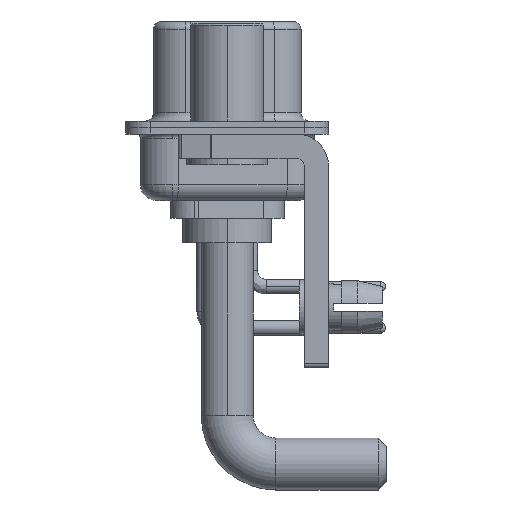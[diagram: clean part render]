
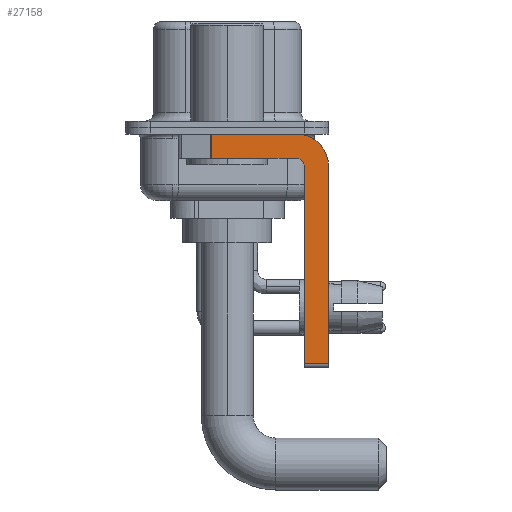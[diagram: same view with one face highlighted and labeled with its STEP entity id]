
A CAD part, left-side view. The second image highlights one B-rep face of the part: STEP entity #27158.
In plain terms, the highlighted planar face has unit normal (-1, 0, 0).
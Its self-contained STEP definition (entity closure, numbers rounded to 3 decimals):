
#80 = AXIS2_PLACEMENT_3D ( 'NONE', #9744, #21357, #2377 ) ;
#564 = VERTEX_POINT ( 'NONE', #26836 ) ;
#746 = VERTEX_POINT ( 'NONE', #25038 ) ;
#824 = DIRECTION ( 'NONE',  ( 0., 0., 1. ) ) ;
#880 = DIRECTION ( 'NONE',  ( 1., 0., 0. ) ) ;
#1668 = CARTESIAN_POINT ( 'NONE',  ( -2.9, -4.75, -14.55 ) ) ;
#2377 = DIRECTION ( 'NONE',  ( 0., 0., -1. ) ) ;
#2420 = DIRECTION ( 'NONE',  ( 0., 0., 1. ) ) ;
#3347 = CARTESIAN_POINT ( 'NONE',  ( -2.9, -6.25, -2.4 ) ) ;
#4554 = LINE ( 'NONE', #18276, #5144 ) ;
#5144 = VECTOR ( 'NONE', #24748, 1000. ) ;
#5225 = VECTOR ( 'NONE', #15103, 1000. ) ;
#5374 = EDGE_CURVE ( 'NONE', #10160, #24818, #15476, .T. ) ;
#5431 = CARTESIAN_POINT ( 'NONE',  ( -2.9, -4.25, -1.9 ) ) ;
#5654 = VERTEX_POINT ( 'NONE', #15479 ) ;
#6019 = EDGE_CURVE ( 'NONE', #564, #11332, #23209, .T. ) ;
#6209 = LINE ( 'NONE', #13156, #9062 ) ;
#7312 = DIRECTION ( 'NONE',  ( 0., 0., -1. ) ) ;
#7563 = ORIENTED_EDGE ( 'NONE', *, *, #7827, .T. ) ;
#7827 = EDGE_CURVE ( 'NONE', #16500, #746, #23149, .T. ) ;
#9062 = VECTOR ( 'NONE', #22341, 1000. ) ;
#9518 = ORIENTED_EDGE ( 'NONE', *, *, #23897, .F. ) ;
#9744 = CARTESIAN_POINT ( 'NONE',  ( -2.9, -4.25, -2.4 ) ) ;
#9854 = ORIENTED_EDGE ( 'NONE', *, *, #5374, .F. ) ;
#10160 = VERTEX_POINT ( 'NONE', #23318 ) ;
#10412 = VECTOR ( 'NONE', #2420, 1000. ) ;
#10636 = ORIENTED_EDGE ( 'NONE', *, *, #24202, .F. ) ;
#11120 = ORIENTED_EDGE ( 'NONE', *, *, #20179, .F. ) ;
#11332 = VERTEX_POINT ( 'NONE', #5431 ) ;
#11655 = AXIS2_PLACEMENT_3D ( 'NONE', #23871, #23416, #824 ) ;
#11969 = ORIENTED_EDGE ( 'NONE', *, *, #23213, .F. ) ;
#13156 = CARTESIAN_POINT ( 'NONE',  ( -2.9, -4.25, -1.9 ) ) ;
#13578 = VERTEX_POINT ( 'NONE', #1668 ) ;
#13690 = CARTESIAN_POINT ( 'NONE',  ( -2.9, 0.978, -0.4 ) ) ;
#13928 = VECTOR ( 'NONE', #7312, 1000. ) ;
#14303 = LINE ( 'NONE', #23504, #10412 ) ;
#14587 = PLANE ( 'NONE',  #27497 ) ;
#14854 = ORIENTED_EDGE ( 'NONE', *, *, #21497, .T. ) ;
#15103 = DIRECTION ( 'NONE',  ( 0., 0., -1. ) ) ;
#15476 = CIRCLE ( 'NONE', #80, 2. ) ;
#15479 = CARTESIAN_POINT ( 'NONE',  ( -2.9, -6.25, -14.55 ) ) ;
#16124 = EDGE_LOOP ( 'NONE', ( #10636, #7563, #11120, #19081, #9518, #14854, #11969, #9854 ) ) ;
#16500 = VERTEX_POINT ( 'NONE', #13690 ) ;
#17644 = LINE ( 'NONE', #3347, #5225 ) ;
#18276 = CARTESIAN_POINT ( 'NONE',  ( -2.9, -4.25, -14.55 ) ) ;
#19081 = ORIENTED_EDGE ( 'NONE', *, *, #6019, .F. ) ;
#19895 = DIRECTION ( 'NONE',  ( 0., -1., 0. ) ) ;
#20179 = EDGE_CURVE ( 'NONE', #11332, #746, #6209, .T. ) ;
#21357 = DIRECTION ( 'NONE',  ( 1., 0., 0. ) ) ;
#21497 = EDGE_CURVE ( 'NONE', #13578, #5654, #4554, .T. ) ;
#22341 = DIRECTION ( 'NONE',  ( 0., 1., 0. ) ) ;
#22572 = VECTOR ( 'NONE', #19895, 1000. ) ;
#23149 = LINE ( 'NONE', #23432, #13928 ) ;
#23209 = CIRCLE ( 'NONE', #11655, 0.5 ) ;
#23213 = EDGE_CURVE ( 'NONE', #24818, #5654, #17644, .T. ) ;
#23318 = CARTESIAN_POINT ( 'NONE',  ( -2.9, -4.25, -0.4 ) ) ;
#23416 = DIRECTION ( 'NONE',  ( -1., 0., 0. ) ) ;
#23432 = CARTESIAN_POINT ( 'NONE',  ( -2.9, 0.978, -1.9 ) ) ;
#23504 = CARTESIAN_POINT ( 'NONE',  ( -2.9, -4.75, -14.8 ) ) ;
#23540 = CARTESIAN_POINT ( 'NONE',  ( -2.9, -6.25, -2.4 ) ) ;
#23778 = DIRECTION ( 'NONE',  ( 0., 0., -1. ) ) ;
#23871 = CARTESIAN_POINT ( 'NONE',  ( -2.9, -4.25, -2.4 ) ) ;
#23897 = EDGE_CURVE ( 'NONE', #13578, #564, #14303, .T. ) ;
#24202 = EDGE_CURVE ( 'NONE', #16500, #10160, #29634, .T. ) ;
#24544 = CARTESIAN_POINT ( 'NONE',  ( -2.9, 3., -0.4 ) ) ;
#24748 = DIRECTION ( 'NONE',  ( 0., -1., 0. ) ) ;
#24818 = VERTEX_POINT ( 'NONE', #23540 ) ;
#25038 = CARTESIAN_POINT ( 'NONE',  ( -2.9, 0.978, -1.9 ) ) ;
#26631 = CARTESIAN_POINT ( 'NONE',  ( -2.9, -4.25, -2.4 ) ) ;
#26836 = CARTESIAN_POINT ( 'NONE',  ( -2.9, -4.75, -2.4 ) ) ;
#27158 = ADVANCED_FACE ( 'NONE', ( #29039 ), #14587, .F. ) ;
#27497 = AXIS2_PLACEMENT_3D ( 'NONE', #26631, #880, #23778 ) ;
#29039 = FACE_OUTER_BOUND ( 'NONE', #16124, .T. ) ;
#29634 = LINE ( 'NONE', #24544, #22572 ) ;
